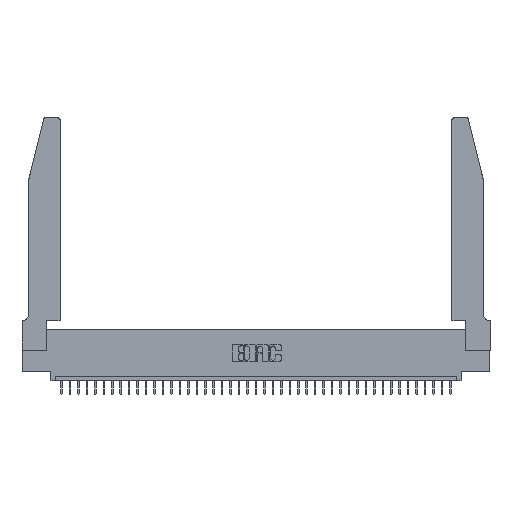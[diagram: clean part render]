
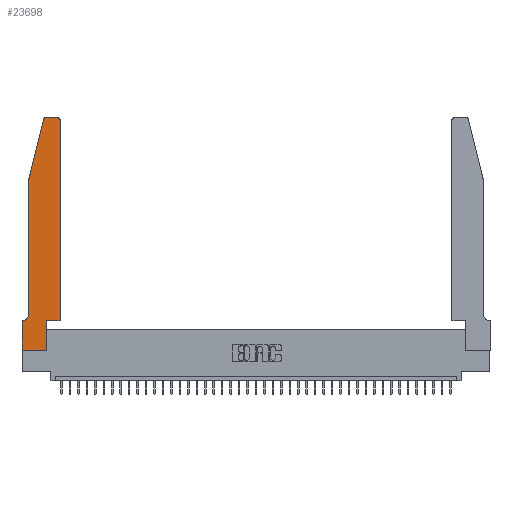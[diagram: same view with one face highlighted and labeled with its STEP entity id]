
A CAD part, top view. The second image highlights one B-rep face of the part: STEP entity #23698.
In plain terms, the highlighted planar face has unit normal (0, 0, 1).
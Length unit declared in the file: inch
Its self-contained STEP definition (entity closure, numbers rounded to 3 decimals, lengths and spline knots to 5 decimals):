
#340 = ORIENTED_EDGE ( 'NONE', *, *, #3438, .T. ) ;
#1586 = LINE ( 'NONE', #19803, #33233 ) ;
#1793 = EDGE_CURVE ( 'NONE', #29519, #13539, #12807, .T. ) ;
#1910 = CARTESIAN_POINT ( 'NONE',  ( 0.4205, 2.72, 0.37 ) ) ;
#2316 = CIRCLE ( 'NONE', #8018, 0.03 ) ;
#2804 = CARTESIAN_POINT ( 'NONE',  ( 0.25487, 2.72718, 0.37 ) ) ;
#3222 = VECTOR ( 'NONE', #22261, 39.37008 ) ;
#3283 = VECTOR ( 'NONE', #14620, 39.37008 ) ;
#3438 = EDGE_CURVE ( 'NONE', #13596, #29519, #7914, .T. ) ;
#3639 = VERTEX_POINT ( 'NONE', #15531 ) ;
#5179 = DIRECTION ( 'NONE',  ( 0., 0., 1. ) ) ;
#5548 = EDGE_CURVE ( 'NONE', #31206, #17220, #15448, .T. ) ;
#6721 = AXIS2_PLACEMENT_3D ( 'NONE', #8291, #5179, #36210 ) ;
#7045 = EDGE_CURVE ( 'NONE', #13539, #24566, #2316, .T. ) ;
#7271 = CARTESIAN_POINT ( 'NONE',  ( 0., 0., 0.37 ) ) ;
#7914 = LINE ( 'NONE', #36155, #39492 ) ;
#7941 = ORIENTED_EDGE ( 'NONE', *, *, #35554, .T. ) ;
#7962 = EDGE_CURVE ( 'NONE', #32029, #13596, #18581, .T. ) ;
#8018 = AXIS2_PLACEMENT_3D ( 'NONE', #1910, #14553, #32606 ) ;
#8260 = DIRECTION ( 'NONE',  ( -1., 0., 0. ) ) ;
#8291 = CARTESIAN_POINT ( 'NONE',  ( 0.284, 2.72, 0.37 ) ) ;
#8795 = AXIS2_PLACEMENT_3D ( 'NONE', #30211, #9722, #24825 ) ;
#9722 = DIRECTION ( 'NONE',  ( 0., 0., 1. ) ) ;
#9980 = ORIENTED_EDGE ( 'NONE', *, *, #5548, .T. ) ;
#9998 = LINE ( 'NONE', #29536, #28687 ) ;
#10049 = VERTEX_POINT ( 'NONE', #31983 ) ;
#10082 = EDGE_CURVE ( 'NONE', #27432, #10310, #1586, .T. ) ;
#10310 = VERTEX_POINT ( 'NONE', #21262 ) ;
#12350 = VECTOR ( 'NONE', #12960, 39.37008 ) ;
#12807 = LINE ( 'NONE', #23486, #30539 ) ;
#12960 = DIRECTION ( 'NONE',  ( 0., 1., 0. ) ) ;
#13190 = CARTESIAN_POINT ( 'NONE',  ( 0.0755, 2., 0.37 ) ) ;
#13470 = EDGE_LOOP ( 'NONE', ( #14474, #9980, #28275, #7941, #14475, #25158, #19953, #30228, #35665, #340, #23806, #21841 ) ) ;
#13539 = VERTEX_POINT ( 'NONE', #33204 ) ;
#13596 = VERTEX_POINT ( 'NONE', #27304 ) ;
#13780 = CARTESIAN_POINT ( 'NONE',  ( 0.284, 2.75, 0.37 ) ) ;
#14474 = ORIENTED_EDGE ( 'NONE', *, *, #38933, .T. ) ;
#14475 = ORIENTED_EDGE ( 'NONE', *, *, #30012, .T. ) ;
#14553 = DIRECTION ( 'NONE',  ( 0., 0., 1. ) ) ;
#14620 = DIRECTION ( 'NONE',  ( -1., 0., 0. ) ) ;
#15448 = CIRCLE ( 'NONE', #6721, 0.03 ) ;
#15531 = CARTESIAN_POINT ( 'NONE',  ( 0.0055, 0.35, 0.37 ) ) ;
#16160 = DIRECTION ( 'NONE',  ( 0., 0., -1. ) ) ;
#17153 = CARTESIAN_POINT ( 'NONE',  ( 0.0755, 2., 0.37 ) ) ;
#17220 = VERTEX_POINT ( 'NONE', #2804 ) ;
#17439 = EDGE_CURVE ( 'NONE', #3639, #27432, #9998, .T. ) ;
#18204 = CARTESIAN_POINT ( 'NONE',  ( 0.2865, 0.35, 0.37 ) ) ;
#18581 = LINE ( 'NONE', #18204, #12350 ) ;
#18683 = DIRECTION ( 'NONE',  ( -1., 0., 0. ) ) ;
#19535 = LINE ( 'NONE', #7271, #3222 ) ;
#19803 = CARTESIAN_POINT ( 'NONE',  ( 0., 0., 0.37 ) ) ;
#19953 = ORIENTED_EDGE ( 'NONE', *, *, #10082, .T. ) ;
#21262 = CARTESIAN_POINT ( 'NONE',  ( 0., 0., 0.37 ) ) ;
#21841 = ORIENTED_EDGE ( 'NONE', *, *, #7045, .T. ) ;
#22261 = DIRECTION ( 'NONE',  ( 1., 0., 0. ) ) ;
#23349 = PLANE ( 'NONE',  #8795 ) ;
#23486 = CARTESIAN_POINT ( 'NONE',  ( 0.4505, 0.35, 0.37 ) ) ;
#23698 = ADVANCED_FACE ( 'NONE', ( #30105 ), #23349, .T. ) ;
#23806 = ORIENTED_EDGE ( 'NONE', *, *, #1793, .T. ) ;
#23971 = EDGE_CURVE ( 'NONE', #10310, #32029, #19535, .T. ) ;
#24566 = VERTEX_POINT ( 'NONE', #37821 ) ;
#24825 = DIRECTION ( 'NONE',  ( 1., 0., 0. ) ) ;
#25158 = ORIENTED_EDGE ( 'NONE', *, *, #17439, .T. ) ;
#25200 = LINE ( 'NONE', #13190, #35251 ) ;
#26069 = DIRECTION ( 'NONE',  ( 0., -1., 0. ) ) ;
#26950 = LINE ( 'NONE', #17153, #33168 ) ;
#27304 = CARTESIAN_POINT ( 'NONE',  ( 0.2865, 0.35, 0.37 ) ) ;
#27346 = DIRECTION ( 'NONE',  ( 1., 0., 0. ) ) ;
#27432 = VERTEX_POINT ( 'NONE', #39574 ) ;
#28275 = ORIENTED_EDGE ( 'NONE', *, *, #31367, .T. ) ;
#28461 = CARTESIAN_POINT ( 'NONE',  ( 0.4505, 0.35, 0.37 ) ) ;
#28687 = VECTOR ( 'NONE', #8260, 39.37008 ) ;
#29519 = VERTEX_POINT ( 'NONE', #28461 ) ;
#29536 = CARTESIAN_POINT ( 'NONE',  ( 0.0755, 0.35, 0.37 ) ) ;
#29860 = CARTESIAN_POINT ( 'NONE',  ( 0.2605, 2.75, 0.37 ) ) ;
#29952 = CIRCLE ( 'NONE', #36287, 0.07 ) ;
#30012 = EDGE_CURVE ( 'NONE', #10049, #3639, #29952, .T. ) ;
#30105 = FACE_OUTER_BOUND ( 'NONE', #13470, .T. ) ;
#30211 = CARTESIAN_POINT ( 'NONE',  ( 0., 0.35, 0.37 ) ) ;
#30228 = ORIENTED_EDGE ( 'NONE', *, *, #23971, .T. ) ;
#30539 = VECTOR ( 'NONE', #39116, 39.37008 ) ;
#31206 = VERTEX_POINT ( 'NONE', #13780 ) ;
#31367 = EDGE_CURVE ( 'NONE', #17220, #36563, #26950, .T. ) ;
#31391 = DIRECTION ( 'NONE',  ( 0., -1., 0. ) ) ;
#31983 = CARTESIAN_POINT ( 'NONE',  ( 0.0755, 0.42, 0.37 ) ) ;
#32029 = VERTEX_POINT ( 'NONE', #38802 ) ;
#32606 = DIRECTION ( 'NONE',  ( 1., 0., 0. ) ) ;
#33168 = VECTOR ( 'NONE', #38852, 39.37008 ) ;
#33204 = CARTESIAN_POINT ( 'NONE',  ( 0.4505, 2.72, 0.37 ) ) ;
#33233 = VECTOR ( 'NONE', #26069, 39.37008 ) ;
#33952 = LINE ( 'NONE', #29860, #3283 ) ;
#34187 = CARTESIAN_POINT ( 'NONE',  ( 0.0055, 0.42, 0.37 ) ) ;
#34239 = CARTESIAN_POINT ( 'NONE',  ( 0.0755, 2., 0.37 ) ) ;
#35251 = VECTOR ( 'NONE', #31391, 39.37008 ) ;
#35554 = EDGE_CURVE ( 'NONE', #36563, #10049, #25200, .T. ) ;
#35665 = ORIENTED_EDGE ( 'NONE', *, *, #7962, .T. ) ;
#36155 = CARTESIAN_POINT ( 'NONE',  ( 0.4505, 0.35, 0.37 ) ) ;
#36210 = DIRECTION ( 'NONE',  ( 1., 0., 0. ) ) ;
#36287 = AXIS2_PLACEMENT_3D ( 'NONE', #34187, #16160, #18683 ) ;
#36563 = VERTEX_POINT ( 'NONE', #34239 ) ;
#37821 = CARTESIAN_POINT ( 'NONE',  ( 0.4205, 2.75, 0.37 ) ) ;
#38802 = CARTESIAN_POINT ( 'NONE',  ( 0.2865, 0., 0.37 ) ) ;
#38852 = DIRECTION ( 'NONE',  ( -0.239, -0.971, 0. ) ) ;
#38933 = EDGE_CURVE ( 'NONE', #24566, #31206, #33952, .T. ) ;
#39116 = DIRECTION ( 'NONE',  ( 0., 1., 0. ) ) ;
#39492 = VECTOR ( 'NONE', #27346, 39.37008 ) ;
#39574 = CARTESIAN_POINT ( 'NONE',  ( 0., 0.35, 0.37 ) ) ;
